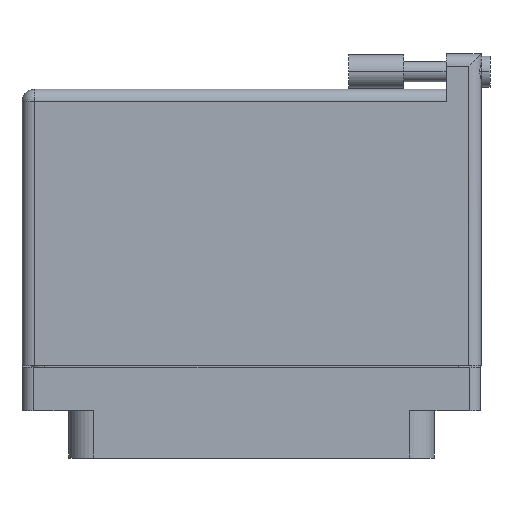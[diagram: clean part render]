
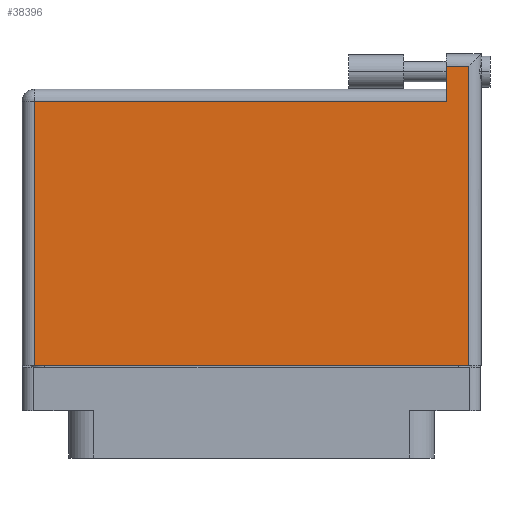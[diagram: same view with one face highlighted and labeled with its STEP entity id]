
A CAD part, front view. The second image highlights one B-rep face of the part: STEP entity #38396.
In plain terms, the highlighted face is planar.
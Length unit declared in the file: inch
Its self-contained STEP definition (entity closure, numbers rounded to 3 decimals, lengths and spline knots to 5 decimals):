
#1150 = ORIENTED_EDGE ( 'NONE', *, *, #26623, .T. ) ;
#2991 = DIRECTION ( 'NONE',  ( 0., -1., 0. ) ) ;
#4719 = DIRECTION ( 'NONE',  ( 0., -1., 0. ) ) ;
#5040 = CARTESIAN_POINT ( 'NONE',  ( 1.103, 1.596, 0.4495 ) ) ;
#5761 = DIRECTION ( 'NONE',  ( 1., 0., 0. ) ) ;
#5830 = VECTOR ( 'NONE', #35429, 39.37008 ) ;
#5919 = CARTESIAN_POINT ( 'NONE',  ( -1.3, 1.596, 0.4495 ) ) ;
#6137 = DIRECTION ( 'NONE',  ( 0., 1., 0. ) ) ;
#7405 = EDGE_CURVE ( 'NONE', #45311, #18532, #12650, .T. ) ;
#9877 = ORIENTED_EDGE ( 'NONE', *, *, #42771, .T. ) ;
#10736 = VERTEX_POINT ( 'NONE', #28285 ) ;
#12171 = CARTESIAN_POINT ( 'NONE',  ( 1.23, 1.596, 0.4495 ) ) ;
#12650 = LINE ( 'NONE', #13402, #40846 ) ;
#13402 = CARTESIAN_POINT ( 'NONE',  ( 1.23, 1.666, 0.4495 ) ) ;
#13675 = CARTESIAN_POINT ( 'NONE',  ( -1.23, 1.396, 0.4495 ) ) ;
#14813 = EDGE_LOOP ( 'NONE', ( #25319, #28661, #9877, #40004, #1150, #34906 ) ) ;
#15652 = LINE ( 'NONE', #16514, #5830 ) ;
#15849 = VERTEX_POINT ( 'NONE', #5040 ) ;
#16327 = LINE ( 'NONE', #27800, #33523 ) ;
#16514 = CARTESIAN_POINT ( 'NONE',  ( -1.3, 1.396, 0.4495 ) ) ;
#18532 = VERTEX_POINT ( 'NONE', #12171 ) ;
#20069 = LINE ( 'NONE', #5919, #22885 ) ;
#21555 = CARTESIAN_POINT ( 'NONE',  ( -1.3, 1.466, 0.4495 ) ) ;
#22885 = VECTOR ( 'NONE', #31161, 39.37008 ) ;
#25038 = DIRECTION ( 'NONE',  ( 0., 0., -1. ) ) ;
#25319 = ORIENTED_EDGE ( 'NONE', *, *, #40400, .T. ) ;
#26623 = EDGE_CURVE ( 'NONE', #10736, #45272, #15652, .T. ) ;
#27257 = EDGE_CURVE ( 'NONE', #15849, #10736, #43131, .T. ) ;
#27800 = CARTESIAN_POINT ( 'NONE',  ( -1.3, -0.1, 0.4495 ) ) ;
#28285 = CARTESIAN_POINT ( 'NONE',  ( 1.103, 1.396, 0.4495 ) ) ;
#28661 = ORIENTED_EDGE ( 'NONE', *, *, #7405, .T. ) ;
#28742 = DIRECTION ( 'NONE',  ( -1., 0., 0. ) ) ;
#29370 = VECTOR ( 'NONE', #2991, 39.37008 ) ;
#30797 = FACE_OUTER_BOUND ( 'NONE', #14813, .T. ) ;
#31161 = DIRECTION ( 'NONE',  ( -1., 0., 0. ) ) ;
#32002 = EDGE_CURVE ( 'NONE', #45272, #33231, #42320, .T. ) ;
#33231 = VERTEX_POINT ( 'NONE', #44340 ) ;
#33523 = VECTOR ( 'NONE', #5761, 39.37008 ) ;
#34906 = ORIENTED_EDGE ( 'NONE', *, *, #32002, .T. ) ;
#35429 = DIRECTION ( 'NONE',  ( -1., 0., 0. ) ) ;
#36813 = CARTESIAN_POINT ( 'NONE',  ( 1.103, 1.666, 0.4495 ) ) ;
#37212 = VECTOR ( 'NONE', #4719, 39.37008 ) ;
#38396 = ADVANCED_FACE ( 'NONE', ( #30797 ), #40064, .F. ) ;
#40004 = ORIENTED_EDGE ( 'NONE', *, *, #27257, .T. ) ;
#40064 = PLANE ( 'NONE',  #41175 ) ;
#40400 = EDGE_CURVE ( 'NONE', #33231, #45311, #16327, .T. ) ;
#40846 = VECTOR ( 'NONE', #6137, 39.37008 ) ;
#41175 = AXIS2_PLACEMENT_3D ( 'NONE', #21555, #25038, #28742 ) ;
#41387 = CARTESIAN_POINT ( 'NONE',  ( -1.23, -0.1, 0.4495 ) ) ;
#42320 = LINE ( 'NONE', #41387, #37212 ) ;
#42594 = CARTESIAN_POINT ( 'NONE',  ( 1.23, -0.1, 0.4495 ) ) ;
#42771 = EDGE_CURVE ( 'NONE', #18532, #15849, #20069, .T. ) ;
#43131 = LINE ( 'NONE', #36813, #29370 ) ;
#44340 = CARTESIAN_POINT ( 'NONE',  ( -1.23, -0.1, 0.4495 ) ) ;
#45272 = VERTEX_POINT ( 'NONE', #13675 ) ;
#45311 = VERTEX_POINT ( 'NONE', #42594 ) ;
